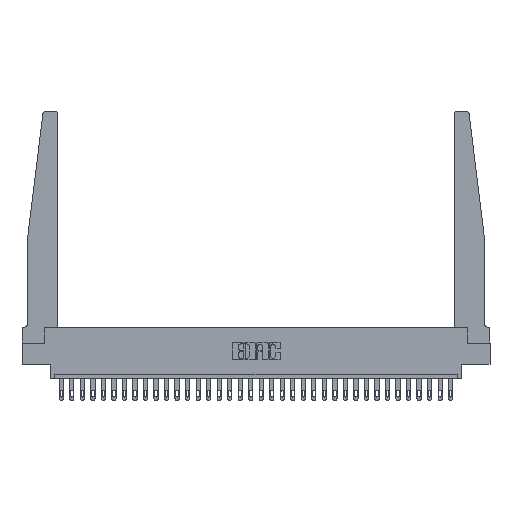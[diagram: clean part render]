
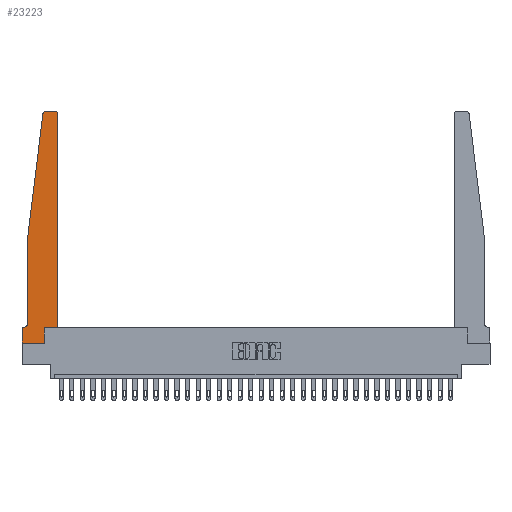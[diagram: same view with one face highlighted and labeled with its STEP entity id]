
A CAD part, top view. The second image highlights one B-rep face of the part: STEP entity #23223.
In plain terms, the highlighted planar face has unit normal (0, 0, 1).
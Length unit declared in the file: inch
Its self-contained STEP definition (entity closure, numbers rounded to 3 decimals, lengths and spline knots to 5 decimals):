
#103 = DIRECTION ( 'NONE',  ( -0.122, -0.992, 0. ) ) ;
#154 = VECTOR ( 'NONE', #14015, 39.37008 ) ;
#189 = ORIENTED_EDGE ( 'NONE', *, *, #17273, .T. ) ;
#223 = ORIENTED_EDGE ( 'NONE', *, *, #1541, .T. ) ;
#325 = DIRECTION ( 'NONE',  ( 1., 0., 0. ) ) ;
#676 = CARTESIAN_POINT ( 'NONE',  ( 0.2605, 0., 0.37 ) ) ;
#918 = CARTESIAN_POINT ( 'NONE',  ( 0.065, 1.25, 0.37 ) ) ;
#1541 = EDGE_CURVE ( 'NONE', #18804, #16056, #12067, .T. ) ;
#1725 = CIRCLE ( 'NONE', #9366, 0.03 ) ;
#2414 = CARTESIAN_POINT ( 'NONE',  ( 0.425, 0.18, 0.37 ) ) ;
#2725 = VERTEX_POINT ( 'NONE', #8654 ) ;
#3363 = CARTESIAN_POINT ( 'NONE',  ( 0.395, 2.75, 0.37 ) ) ;
#4498 = DIRECTION ( 'NONE',  ( 0., 1., 0. ) ) ;
#4734 = EDGE_CURVE ( 'NONE', #16056, #23923, #16001, .T. ) ;
#4816 = LINE ( 'NONE', #13890, #20018 ) ;
#5086 = VECTOR ( 'NONE', #8703, 39.37008 ) ;
#5400 = EDGE_CURVE ( 'NONE', #21280, #18804, #23144, .T. ) ;
#5569 = ORIENTED_EDGE ( 'NONE', *, *, #8422, .T. ) ;
#6708 = CARTESIAN_POINT ( 'NONE',  ( 0.25, 2.75, 0.37 ) ) ;
#6790 = ORIENTED_EDGE ( 'NONE', *, *, #8490, .T. ) ;
#6797 = EDGE_CURVE ( 'NONE', #23452, #17435, #22577, .T. ) ;
#6951 = VECTOR ( 'NONE', #103, 39.37008 ) ;
#7020 = AXIS2_PLACEMENT_3D ( 'NONE', #21248, #19031, #16797 ) ;
#7069 = CARTESIAN_POINT ( 'NONE',  ( 0., 0., 0.37 ) ) ;
#7369 = CARTESIAN_POINT ( 'NONE',  ( 0.24675, 2.72367, 0.37 ) ) ;
#8109 = AXIS2_PLACEMENT_3D ( 'NONE', #12467, #19301, #18741 ) ;
#8158 = CARTESIAN_POINT ( 'NONE',  ( 0.27653, 2.72, 0.37 ) ) ;
#8422 = EDGE_CURVE ( 'NONE', #28426, #23452, #4816, .T. ) ;
#8490 = EDGE_CURVE ( 'NONE', #11882, #21280, #19210, .T. ) ;
#8654 = CARTESIAN_POINT ( 'NONE',  ( 0.27653, 2.75, 0.37 ) ) ;
#8703 = DIRECTION ( 'NONE',  ( 0., -1., 0. ) ) ;
#8858 = LINE ( 'NONE', #10800, #29301 ) ;
#8945 = LINE ( 'NONE', #6708, #10877 ) ;
#9346 = DIRECTION ( 'NONE',  ( 0., 1., 0. ) ) ;
#9366 = AXIS2_PLACEMENT_3D ( 'NONE', #8158, #10116, #26136 ) ;
#9981 = EDGE_CURVE ( 'NONE', #20313, #2725, #8945, .T. ) ;
#10116 = DIRECTION ( 'NONE',  ( 0., 0., 1. ) ) ;
#10146 = ORIENTED_EDGE ( 'NONE', *, *, #16725, .T. ) ;
#10286 = DIRECTION ( 'NONE',  ( 0., -1., 0. ) ) ;
#10800 = CARTESIAN_POINT ( 'NONE',  ( 0., 0., 0.37 ) ) ;
#10877 = VECTOR ( 'NONE', #22019, 39.37008 ) ;
#10971 = CIRCLE ( 'NONE', #8109, 0.03 ) ;
#11834 = VECTOR ( 'NONE', #10286, 39.37008 ) ;
#11882 = VERTEX_POINT ( 'NONE', #22954 ) ;
#12067 = LINE ( 'NONE', #18319, #154 ) ;
#12278 = ORIENTED_EDGE ( 'NONE', *, *, #22545, .T. ) ;
#12467 = CARTESIAN_POINT ( 'NONE',  ( 0.395, 2.72, 0.37 ) ) ;
#12536 = CARTESIAN_POINT ( 'NONE',  ( 0.2605, 0.18, 0.37 ) ) ;
#12617 = EDGE_LOOP ( 'NONE', ( #26731, #10146, #19845, #6790, #23587, #223, #23902, #189, #20290, #5569, #12791, #12278 ) ) ;
#12791 = ORIENTED_EDGE ( 'NONE', *, *, #6797, .T. ) ;
#13890 = CARTESIAN_POINT ( 'NONE',  ( 0.425, 0.18, 0.37 ) ) ;
#14015 = DIRECTION ( 'NONE',  ( -1., 0., 0. ) ) ;
#15760 = CARTESIAN_POINT ( 'NONE',  ( 0.425, 0.18, 0.37 ) ) ;
#15788 = EDGE_CURVE ( 'NONE', #18635, #11882, #18562, .T. ) ;
#15965 = CARTESIAN_POINT ( 'NONE',  ( 0., 0.1875, 0.37 ) ) ;
#16001 = LINE ( 'NONE', #7069, #5086 ) ;
#16056 = VERTEX_POINT ( 'NONE', #15965 ) ;
#16725 = EDGE_CURVE ( 'NONE', #2725, #18635, #1725, .T. ) ;
#16797 = DIRECTION ( 'NONE',  ( -1., 0., 0. ) ) ;
#17273 = EDGE_CURVE ( 'NONE', #23923, #27825, #8858, .T. ) ;
#17435 = VERTEX_POINT ( 'NONE', #23417 ) ;
#17481 = DIRECTION ( 'NONE',  ( 1., 0., 0. ) ) ;
#18207 = CARTESIAN_POINT ( 'NONE',  ( 0.015, 0.1875, 0.37 ) ) ;
#18319 = CARTESIAN_POINT ( 'NONE',  ( 0.065, 0.1875, 0.37 ) ) ;
#18562 = LINE ( 'NONE', #20505, #6951 ) ;
#18635 = VERTEX_POINT ( 'NONE', #7369 ) ;
#18741 = DIRECTION ( 'NONE',  ( 1., 0., 0. ) ) ;
#18804 = VERTEX_POINT ( 'NONE', #18207 ) ;
#19031 = DIRECTION ( 'NONE',  ( 0., 0., -1. ) ) ;
#19210 = LINE ( 'NONE', #918, #11834 ) ;
#19301 = DIRECTION ( 'NONE',  ( 0., 0., 1. ) ) ;
#19845 = ORIENTED_EDGE ( 'NONE', *, *, #15788, .T. ) ;
#20010 = DIRECTION ( 'NONE',  ( 1., 0., 0. ) ) ;
#20018 = VECTOR ( 'NONE', #325, 39.37008 ) ;
#20290 = ORIENTED_EDGE ( 'NONE', *, *, #27305, .T. ) ;
#20313 = VERTEX_POINT ( 'NONE', #3363 ) ;
#20425 = LINE ( 'NONE', #28059, #23415 ) ;
#20505 = CARTESIAN_POINT ( 'NONE',  ( 0.065, 1.25, 0.37 ) ) ;
#21248 = CARTESIAN_POINT ( 'NONE',  ( 0.015, 0.2375, 0.37 ) ) ;
#21280 = VERTEX_POINT ( 'NONE', #25255 ) ;
#22019 = DIRECTION ( 'NONE',  ( -1., 0., 0. ) ) ;
#22171 = CARTESIAN_POINT ( 'NONE',  ( 0., 0., 0.37 ) ) ;
#22530 = CARTESIAN_POINT ( 'NONE',  ( 0., 0.1875, 0.37 ) ) ;
#22545 = EDGE_CURVE ( 'NONE', #17435, #20313, #10971, .T. ) ;
#22577 = LINE ( 'NONE', #15760, #22844 ) ;
#22844 = VECTOR ( 'NONE', #9346, 39.37008 ) ;
#22954 = CARTESIAN_POINT ( 'NONE',  ( 0.065, 1.25, 0.37 ) ) ;
#23144 = CIRCLE ( 'NONE', #7020, 0.05 ) ;
#23223 = ADVANCED_FACE ( 'NONE', ( #29039 ), #25189, .T. ) ;
#23415 = VECTOR ( 'NONE', #4498, 39.37008 ) ;
#23417 = CARTESIAN_POINT ( 'NONE',  ( 0.425, 2.72, 0.37 ) ) ;
#23452 = VERTEX_POINT ( 'NONE', #2414 ) ;
#23587 = ORIENTED_EDGE ( 'NONE', *, *, #5400, .T. ) ;
#23902 = ORIENTED_EDGE ( 'NONE', *, *, #4734, .T. ) ;
#23923 = VERTEX_POINT ( 'NONE', #22171 ) ;
#24899 = DIRECTION ( 'NONE',  ( 0., 0., 1. ) ) ;
#25189 = PLANE ( 'NONE',  #28531 ) ;
#25255 = CARTESIAN_POINT ( 'NONE',  ( 0.065, 0.2375, 0.37 ) ) ;
#26136 = DIRECTION ( 'NONE',  ( 1., 0., 0. ) ) ;
#26731 = ORIENTED_EDGE ( 'NONE', *, *, #9981, .T. ) ;
#27305 = EDGE_CURVE ( 'NONE', #27825, #28426, #20425, .T. ) ;
#27825 = VERTEX_POINT ( 'NONE', #676 ) ;
#28059 = CARTESIAN_POINT ( 'NONE',  ( 0.2605, 0.18, 0.37 ) ) ;
#28426 = VERTEX_POINT ( 'NONE', #12536 ) ;
#28531 = AXIS2_PLACEMENT_3D ( 'NONE', #22530, #24899, #20010 ) ;
#29039 = FACE_OUTER_BOUND ( 'NONE', #12617, .T. ) ;
#29301 = VECTOR ( 'NONE', #17481, 39.37008 ) ;
